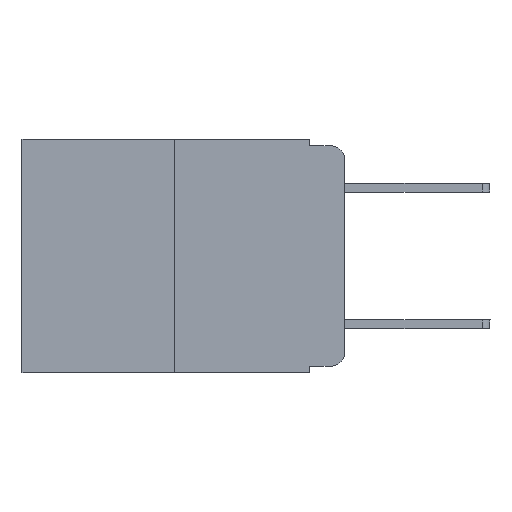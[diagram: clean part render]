
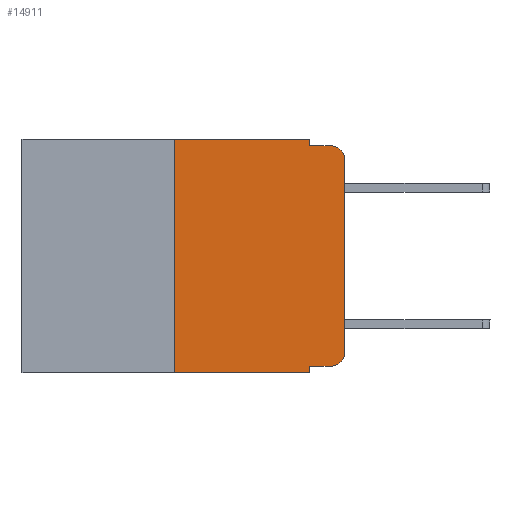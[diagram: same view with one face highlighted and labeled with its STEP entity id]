
A CAD part, left-side view. The second image highlights one B-rep face of the part: STEP entity #14911.
In plain terms, the highlighted planar face has unit normal (-1, 0, 0).
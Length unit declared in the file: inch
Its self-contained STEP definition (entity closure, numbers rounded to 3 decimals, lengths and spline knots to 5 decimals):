
#427 = DIRECTION ( 'NONE',  ( 0., 0., -1. ) ) ;
#502 = CARTESIAN_POINT ( 'NONE',  ( 0., 0.25, -0.343 ) ) ;
#856 = VECTOR ( 'NONE', #19246, 39.37008 ) ;
#966 = CARTESIAN_POINT ( 'NONE',  ( 0., 0., -0.03 ) ) ;
#990 = DIRECTION ( 'NONE',  ( 0., -1., 0. ) ) ;
#1015 = VECTOR ( 'NONE', #15411, 39.37008 ) ;
#1053 = VERTEX_POINT ( 'NONE', #9828 ) ;
#1202 = ORIENTED_EDGE ( 'NONE', *, *, #12759, .T. ) ;
#1529 = DIRECTION ( 'NONE',  ( 0., -1., 0. ) ) ;
#2224 = CARTESIAN_POINT ( 'NONE',  ( 0., 0.02, -0.01 ) ) ;
#2350 = VECTOR ( 'NONE', #990, 39.37008 ) ;
#2706 = AXIS2_PLACEMENT_3D ( 'NONE', #9895, #18857, #9694 ) ;
#2723 = ORIENTED_EDGE ( 'NONE', *, *, #11875, .T. ) ;
#3217 = VERTEX_POINT ( 'NONE', #17475 ) ;
#3449 = CARTESIAN_POINT ( 'NONE',  ( 0., 0.473, 0. ) ) ;
#3518 = CARTESIAN_POINT ( 'NONE',  ( 0., 0.051, 0. ) ) ;
#3767 = LINE ( 'NONE', #18224, #18975 ) ;
#3817 = ORIENTED_EDGE ( 'NONE', *, *, #17905, .T. ) ;
#3872 = VERTEX_POINT ( 'NONE', #8281 ) ;
#3987 = EDGE_CURVE ( 'NONE', #11256, #4096, #16313, .T. ) ;
#4096 = VERTEX_POINT ( 'NONE', #13319 ) ;
#4416 = VECTOR ( 'NONE', #5117, 39.37008 ) ;
#4526 = ORIENTED_EDGE ( 'NONE', *, *, #16183, .T. ) ;
#4681 = VERTEX_POINT ( 'NONE', #7476 ) ;
#5117 = DIRECTION ( 'NONE',  ( 0., 0., 1. ) ) ;
#5312 = ORIENTED_EDGE ( 'NONE', *, *, #3987, .F. ) ;
#5881 = LINE ( 'NONE', #3518, #13465 ) ;
#5965 = EDGE_LOOP ( 'NONE', ( #4526, #3817, #15632, #5312, #13765, #12069, #1202, #8116, #2723, #10460 ) ) ;
#6138 = LINE ( 'NONE', #8724, #2350 ) ;
#6848 = CARTESIAN_POINT ( 'NONE',  ( 0., 0., 0. ) ) ;
#6917 = DIRECTION ( 'NONE',  ( 0., 0., -1. ) ) ;
#7476 = CARTESIAN_POINT ( 'NONE',  ( 0., 0.051, -0.333 ) ) ;
#7515 = EDGE_CURVE ( 'NONE', #19204, #3872, #12368, .T. ) ;
#7520 = AXIS2_PLACEMENT_3D ( 'NONE', #14352, #17477, #6917 ) ;
#8116 = ORIENTED_EDGE ( 'NONE', *, *, #14915, .F. ) ;
#8281 = CARTESIAN_POINT ( 'NONE',  ( 0., 0., -0.313 ) ) ;
#8450 = LINE ( 'NONE', #6848, #4416 ) ;
#8724 = CARTESIAN_POINT ( 'NONE',  ( 0., 0.051, -0.01 ) ) ;
#8777 = CIRCLE ( 'NONE', #2706, 0.02 ) ;
#9694 = DIRECTION ( 'NONE',  ( 0., 0., -1. ) ) ;
#9828 = CARTESIAN_POINT ( 'NONE',  ( 0., 0.25, 0. ) ) ;
#9895 = CARTESIAN_POINT ( 'NONE',  ( 0., 0.02, -0.03 ) ) ;
#10033 = VECTOR ( 'NONE', #15293, 39.37008 ) ;
#10237 = DIRECTION ( 'NONE',  ( 0., -1., 0. ) ) ;
#10375 = CARTESIAN_POINT ( 'NONE',  ( 0., 0.051, -0.333 ) ) ;
#10460 = ORIENTED_EDGE ( 'NONE', *, *, #7515, .T. ) ;
#10988 = CARTESIAN_POINT ( 'NONE',  ( 0., 0.051, 0. ) ) ;
#11256 = VERTEX_POINT ( 'NONE', #10988 ) ;
#11601 = EDGE_CURVE ( 'NONE', #12848, #1053, #18847, .T. ) ;
#11875 = EDGE_CURVE ( 'NONE', #4681, #19204, #15506, .T. ) ;
#12069 = ORIENTED_EDGE ( 'NONE', *, *, #11601, .F. ) ;
#12368 = CIRCLE ( 'NONE', #7520, 0.02 ) ;
#12759 = EDGE_CURVE ( 'NONE', #12848, #3217, #15953, .T. ) ;
#12848 = VERTEX_POINT ( 'NONE', #502 ) ;
#13319 = CARTESIAN_POINT ( 'NONE',  ( 0., 0.051, -0.01 ) ) ;
#13465 = VECTOR ( 'NONE', #427, 39.37008 ) ;
#13765 = ORIENTED_EDGE ( 'NONE', *, *, #17683, .F. ) ;
#13808 = CARTESIAN_POINT ( 'NONE',  ( 0., 0.473, -0.343 ) ) ;
#13833 = VECTOR ( 'NONE', #10237, 39.37008 ) ;
#13954 = FACE_OUTER_BOUND ( 'NONE', #5965, .T. ) ;
#14059 = DIRECTION ( 'NONE',  ( 1., 0., 0. ) ) ;
#14352 = CARTESIAN_POINT ( 'NONE',  ( 0., 0.02, -0.313 ) ) ;
#14411 = EDGE_CURVE ( 'NONE', #4096, #18551, #6138, .T. ) ;
#14911 = ADVANCED_FACE ( 'NONE', ( #13954 ), #17186, .F. ) ;
#14915 = EDGE_CURVE ( 'NONE', #4681, #3217, #5881, .T. ) ;
#15209 = VERTEX_POINT ( 'NONE', #966 ) ;
#15293 = DIRECTION ( 'NONE',  ( 0., -1., 0. ) ) ;
#15350 = CARTESIAN_POINT ( 'NONE',  ( 0., 0.25, 0. ) ) ;
#15411 = DIRECTION ( 'NONE',  ( 0., 0., 1. ) ) ;
#15506 = LINE ( 'NONE', #10375, #13833 ) ;
#15607 = DIRECTION ( 'NONE',  ( 0., 0., -1. ) ) ;
#15632 = ORIENTED_EDGE ( 'NONE', *, *, #14411, .F. ) ;
#15953 = LINE ( 'NONE', #13808, #10033 ) ;
#16183 = EDGE_CURVE ( 'NONE', #3872, #15209, #8450, .T. ) ;
#16191 = CARTESIAN_POINT ( 'NONE',  ( 0., 0.051, 0. ) ) ;
#16313 = LINE ( 'NONE', #16191, #856 ) ;
#17186 = PLANE ( 'NONE',  #17677 ) ;
#17406 = CARTESIAN_POINT ( 'NONE',  ( 0., 0.02, -0.333 ) ) ;
#17475 = CARTESIAN_POINT ( 'NONE',  ( 0., 0.051, -0.343 ) ) ;
#17477 = DIRECTION ( 'NONE',  ( -1., 0., 0. ) ) ;
#17677 = AXIS2_PLACEMENT_3D ( 'NONE', #3449, #14059, #15607 ) ;
#17683 = EDGE_CURVE ( 'NONE', #1053, #11256, #3767, .T. ) ;
#17905 = EDGE_CURVE ( 'NONE', #15209, #18551, #8777, .T. ) ;
#18224 = CARTESIAN_POINT ( 'NONE',  ( 0., 0.473, 0. ) ) ;
#18551 = VERTEX_POINT ( 'NONE', #2224 ) ;
#18847 = LINE ( 'NONE', #15350, #1015 ) ;
#18857 = DIRECTION ( 'NONE',  ( -1., 0., 0. ) ) ;
#18975 = VECTOR ( 'NONE', #1529, 39.37008 ) ;
#19204 = VERTEX_POINT ( 'NONE', #17406 ) ;
#19246 = DIRECTION ( 'NONE',  ( 0., 0., -1. ) ) ;
